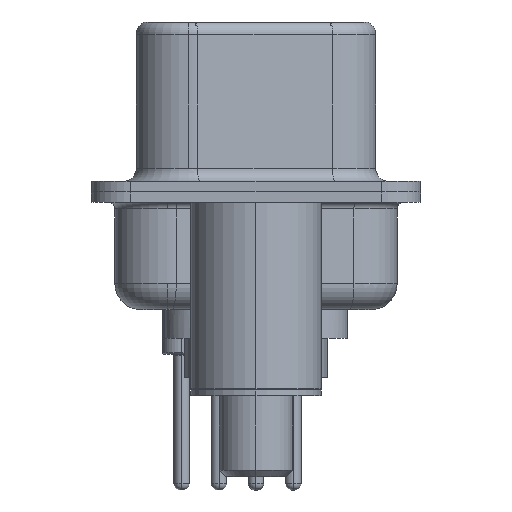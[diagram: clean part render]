
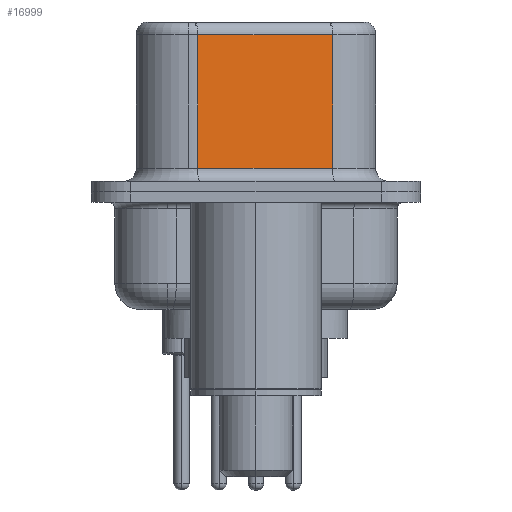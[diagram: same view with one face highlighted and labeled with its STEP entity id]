
A CAD part, left-side view. The second image highlights one B-rep face of the part: STEP entity #16999.
In plain terms, the highlighted planar face has unit normal (-0.985, -0.174, 0).
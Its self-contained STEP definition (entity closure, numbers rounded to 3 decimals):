
#163 = CARTESIAN_POINT ( 'NONE',  ( 4.58, -2.927, 0.9 ) ) ;
#1834 = CARTESIAN_POINT ( 'NONE',  ( 3.67, 2.233, 0.9 ) ) ;
#1981 = DIRECTION ( 'NONE',  ( 0.174, -0.985, 0. ) ) ;
#2289 = VERTEX_POINT ( 'NONE', #1834 ) ;
#2766 = DIRECTION ( 'NONE',  ( 0., 0., -1. ) ) ;
#3530 = EDGE_CURVE ( 'NONE', #15918, #19644, #5845, .T. ) ;
#4064 = FACE_OUTER_BOUND ( 'NONE', #21771, .T. ) ;
#4618 = VECTOR ( 'NONE', #20380, 1000. ) ;
#4622 = DIRECTION ( 'NONE',  ( 0.985, 0.174, 0. ) ) ;
#5023 = CARTESIAN_POINT ( 'NONE',  ( 4.58, -2.927, 6.02 ) ) ;
#5052 = AXIS2_PLACEMENT_3D ( 'NONE', #15394, #4622, #17199 ) ;
#5460 = EDGE_CURVE ( 'NONE', #20011, #2289, #12513, .T. ) ;
#5845 = LINE ( 'NONE', #7183, #10085 ) ;
#5975 = LINE ( 'NONE', #19917, #20827 ) ;
#6323 = PLANE ( 'NONE',  #5052 ) ;
#6693 = EDGE_CURVE ( 'NONE', #2289, #19644, #5975, .T. ) ;
#7183 = CARTESIAN_POINT ( 'NONE',  ( 4.58, -2.927, 6.52 ) ) ;
#7739 = ORIENTED_EDGE ( 'NONE', *, *, #5460, .T. ) ;
#7771 = VECTOR ( 'NONE', #2766, 1000. ) ;
#8665 = ORIENTED_EDGE ( 'NONE', *, *, #22218, .T. ) ;
#9395 = LINE ( 'NONE', #18597, #4618 ) ;
#10085 = VECTOR ( 'NONE', #19797, 1000. ) ;
#10930 = ORIENTED_EDGE ( 'NONE', *, *, #6693, .T. ) ;
#12355 = ORIENTED_EDGE ( 'NONE', *, *, #3530, .F. ) ;
#12513 = LINE ( 'NONE', #16192, #7771 ) ;
#15394 = CARTESIAN_POINT ( 'NONE',  ( 4.58, -2.927, 6.52 ) ) ;
#15918 = VERTEX_POINT ( 'NONE', #5023 ) ;
#16192 = CARTESIAN_POINT ( 'NONE',  ( 3.67, 2.233, 6.52 ) ) ;
#16999 = ADVANCED_FACE ( 'NONE', ( #4064 ), #6323, .F. ) ;
#17199 = DIRECTION ( 'NONE',  ( -0.174, 0.985, 0. ) ) ;
#17790 = CARTESIAN_POINT ( 'NONE',  ( 3.67, 2.233, 6.02 ) ) ;
#18597 = CARTESIAN_POINT ( 'NONE',  ( 4.58, -2.927, 6.02 ) ) ;
#19644 = VERTEX_POINT ( 'NONE', #163 ) ;
#19797 = DIRECTION ( 'NONE',  ( 0., 0., -1. ) ) ;
#19917 = CARTESIAN_POINT ( 'NONE',  ( 4.58, -2.927, 0.9 ) ) ;
#20011 = VERTEX_POINT ( 'NONE', #17790 ) ;
#20380 = DIRECTION ( 'NONE',  ( -0.174, 0.985, 0. ) ) ;
#20827 = VECTOR ( 'NONE', #1981, 1000. ) ;
#21771 = EDGE_LOOP ( 'NONE', ( #12355, #8665, #7739, #10930 ) ) ;
#22218 = EDGE_CURVE ( 'NONE', #15918, #20011, #9395, .T. ) ;
